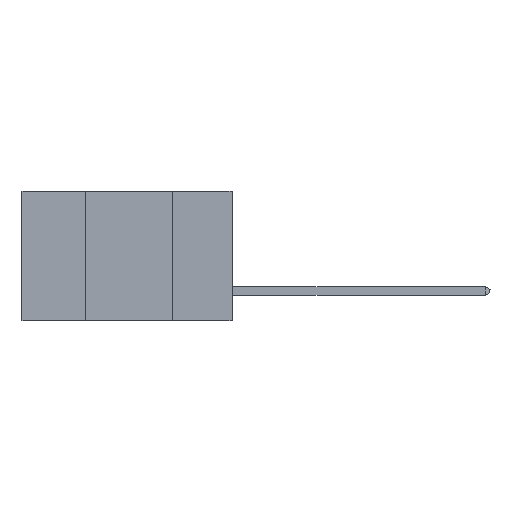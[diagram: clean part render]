
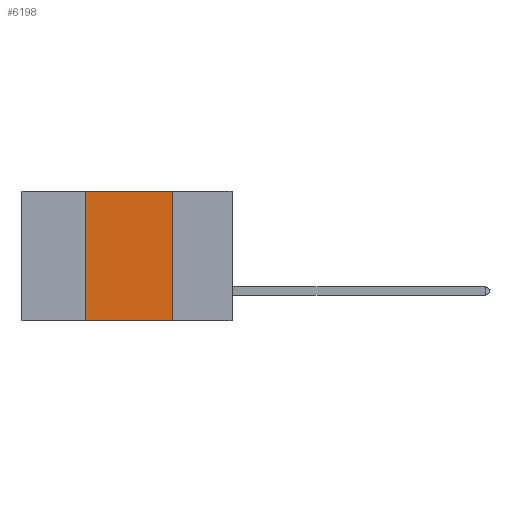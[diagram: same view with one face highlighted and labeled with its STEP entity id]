
A CAD part, left-side view. The second image highlights one B-rep face of the part: STEP entity #6198.
In plain terms, the highlighted planar face has unit normal (-1, 0, 0).
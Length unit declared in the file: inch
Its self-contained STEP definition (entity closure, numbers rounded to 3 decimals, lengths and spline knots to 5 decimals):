
#879 = FACE_OUTER_BOUND ( 'NONE', #12474, .T. ) ;
#1072 = CARTESIAN_POINT ( 'NONE',  ( 0., 0.42, -0.37 ) ) ;
#1149 = EDGE_CURVE ( 'NONE', #9922, #3437, #1209, .T. ) ;
#1209 = LINE ( 'NONE', #3362, #7978 ) ;
#1592 = PLANE ( 'NONE',  #11877 ) ;
#1746 = EDGE_CURVE ( 'NONE', #3437, #5254, #9633, .T. ) ;
#1763 = EDGE_CURVE ( 'NONE', #5908, #5254, #3815, .T. ) ;
#2010 = CARTESIAN_POINT ( 'NONE',  ( 0., 0.42, 0. ) ) ;
#3362 = CARTESIAN_POINT ( 'NONE',  ( 0., 0.6, 0. ) ) ;
#3437 = VERTEX_POINT ( 'NONE', #8140 ) ;
#3815 = LINE ( 'NONE', #9332, #10400 ) ;
#4650 = EDGE_CURVE ( 'NONE', #5908, #9922, #6303, .T. ) ;
#5163 = DIRECTION ( 'NONE',  ( 0., 0., 1. ) ) ;
#5254 = VERTEX_POINT ( 'NONE', #7180 ) ;
#5464 = DIRECTION ( 'NONE',  ( 0., -1., 0. ) ) ;
#5558 = DIRECTION ( 'NONE',  ( 0., 0., -1. ) ) ;
#5908 = VERTEX_POINT ( 'NONE', #1072 ) ;
#6003 = VECTOR ( 'NONE', #5163, 39.37008 ) ;
#6198 = ADVANCED_FACE ( 'NONE', ( #879 ), #1592, .F. ) ;
#6303 = LINE ( 'NONE', #2010, #6003 ) ;
#7089 = ORIENTED_EDGE ( 'NONE', *, *, #1149, .F. ) ;
#7180 = CARTESIAN_POINT ( 'NONE',  ( 0., 0.17, -0.37 ) ) ;
#7978 = VECTOR ( 'NONE', #5464, 39.37008 ) ;
#8072 = CARTESIAN_POINT ( 'NONE',  ( 0., 0.17, 0. ) ) ;
#8113 = DIRECTION ( 'NONE',  ( 0., 0., -1. ) ) ;
#8140 = CARTESIAN_POINT ( 'NONE',  ( 0., 0.17, 0. ) ) ;
#9047 = ORIENTED_EDGE ( 'NONE', *, *, #1746, .F. ) ;
#9332 = CARTESIAN_POINT ( 'NONE',  ( 0., 0.6, -0.37 ) ) ;
#9505 = DIRECTION ( 'NONE',  ( 1., 0., 0. ) ) ;
#9633 = LINE ( 'NONE', #8072, #12347 ) ;
#9922 = VERTEX_POINT ( 'NONE', #11328 ) ;
#10400 = VECTOR ( 'NONE', #10795, 39.37008 ) ;
#10499 = CARTESIAN_POINT ( 'NONE',  ( 0., 0.6, 0. ) ) ;
#10795 = DIRECTION ( 'NONE',  ( 0., -1., 0. ) ) ;
#11271 = ORIENTED_EDGE ( 'NONE', *, *, #4650, .F. ) ;
#11328 = CARTESIAN_POINT ( 'NONE',  ( 0., 0.42, 0. ) ) ;
#11369 = ORIENTED_EDGE ( 'NONE', *, *, #1763, .T. ) ;
#11877 = AXIS2_PLACEMENT_3D ( 'NONE', #10499, #9505, #5558 ) ;
#12347 = VECTOR ( 'NONE', #8113, 39.37008 ) ;
#12474 = EDGE_LOOP ( 'NONE', ( #9047, #7089, #11271, #11369 ) ) ;
